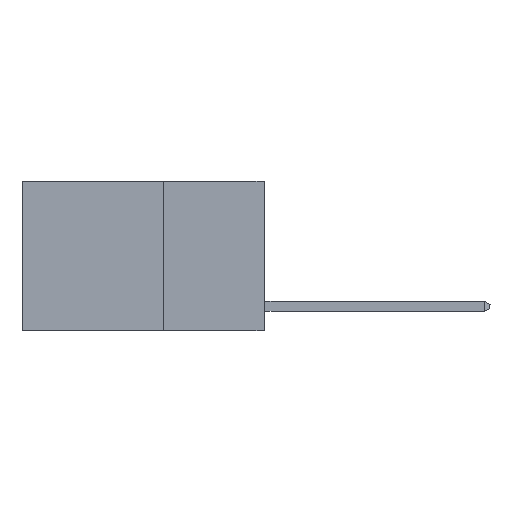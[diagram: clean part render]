
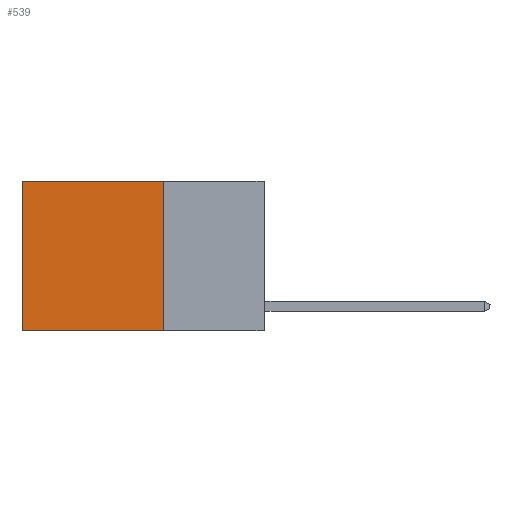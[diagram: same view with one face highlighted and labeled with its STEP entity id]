
A CAD part, left-side view. The second image highlights one B-rep face of the part: STEP entity #539.
In plain terms, the highlighted planar face has unit normal (-1, 0, 0).
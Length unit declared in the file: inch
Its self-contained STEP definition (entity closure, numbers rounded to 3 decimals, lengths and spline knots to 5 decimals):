
#539 = ADVANCED_FACE ( 'NONE', ( #14333 ), #5752, .F. ) ;
#2057 = EDGE_LOOP ( 'NONE', ( #14851, #6419, #29074, #23904 ) ) ;
#2708 = EDGE_CURVE ( 'NONE', #13879, #18724, #26737, .T. ) ;
#3475 = DIRECTION ( 'NONE',  ( 1., 0., 0. ) ) ;
#4235 = CARTESIAN_POINT ( 'NONE',  ( 0.2625, 0.6, 0. ) ) ;
#4262 = EDGE_CURVE ( 'NONE', #18724, #16449, #12236, .T. ) ;
#5752 = PLANE ( 'NONE',  #18397 ) ;
#6419 = ORIENTED_EDGE ( 'NONE', *, *, #4262, .F. ) ;
#6642 = CARTESIAN_POINT ( 'NONE',  ( 0.2625, 0.25, -0.37 ) ) ;
#8657 = LINE ( 'NONE', #14608, #21239 ) ;
#10784 = VERTEX_POINT ( 'NONE', #4235 ) ;
#11169 = CARTESIAN_POINT ( 'NONE',  ( 0.2625, 0.25, -0.37 ) ) ;
#11476 = VECTOR ( 'NONE', #25589, 39.37008 ) ;
#12236 = LINE ( 'NONE', #6642, #11476 ) ;
#12453 = DIRECTION ( 'NONE',  ( 0., 0., -1. ) ) ;
#13023 = EDGE_CURVE ( 'NONE', #10784, #16449, #8657, .T. ) ;
#13879 = VERTEX_POINT ( 'NONE', #20029 ) ;
#14333 = FACE_OUTER_BOUND ( 'NONE', #2057, .T. ) ;
#14472 = DIRECTION ( 'NONE',  ( 0., 1., 0. ) ) ;
#14608 = CARTESIAN_POINT ( 'NONE',  ( 0.2625, 0.6, 0. ) ) ;
#14851 = ORIENTED_EDGE ( 'NONE', *, *, #13023, .T. ) ;
#15490 = EDGE_CURVE ( 'NONE', #13879, #10784, #19960, .T. ) ;
#16449 = VERTEX_POINT ( 'NONE', #22683 ) ;
#18397 = AXIS2_PLACEMENT_3D ( 'NONE', #27074, #3475, #20046 ) ;
#18724 = VERTEX_POINT ( 'NONE', #11169 ) ;
#19218 = VECTOR ( 'NONE', #14472, 39.37008 ) ;
#19552 = CARTESIAN_POINT ( 'NONE',  ( 0.2625, 0.25, 0. ) ) ;
#19960 = LINE ( 'NONE', #21481, #19218 ) ;
#20029 = CARTESIAN_POINT ( 'NONE',  ( 0.2625, 0.25, 0. ) ) ;
#20046 = DIRECTION ( 'NONE',  ( 0., 0., -1. ) ) ;
#20461 = VECTOR ( 'NONE', #12453, 39.37008 ) ;
#21239 = VECTOR ( 'NONE', #21629, 39.37008 ) ;
#21481 = CARTESIAN_POINT ( 'NONE',  ( 0.2625, 0.25, 0. ) ) ;
#21629 = DIRECTION ( 'NONE',  ( 0., 0., -1. ) ) ;
#22683 = CARTESIAN_POINT ( 'NONE',  ( 0.2625, 0.6, -0.37 ) ) ;
#23904 = ORIENTED_EDGE ( 'NONE', *, *, #15490, .T. ) ;
#25589 = DIRECTION ( 'NONE',  ( 0., 1., 0. ) ) ;
#26737 = LINE ( 'NONE', #19552, #20461 ) ;
#27074 = CARTESIAN_POINT ( 'NONE',  ( 0.2625, 0.25, 0. ) ) ;
#29074 = ORIENTED_EDGE ( 'NONE', *, *, #2708, .F. ) ;
